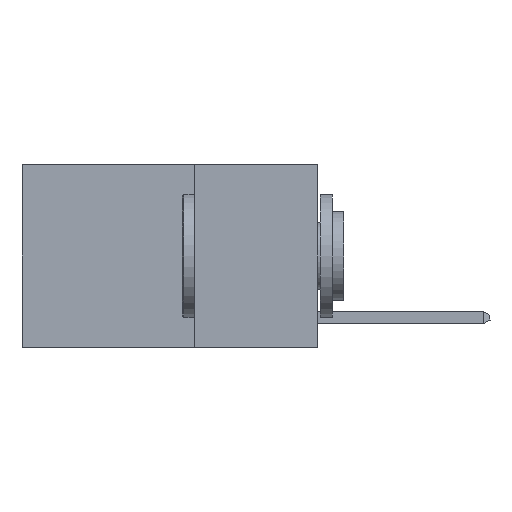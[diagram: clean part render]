
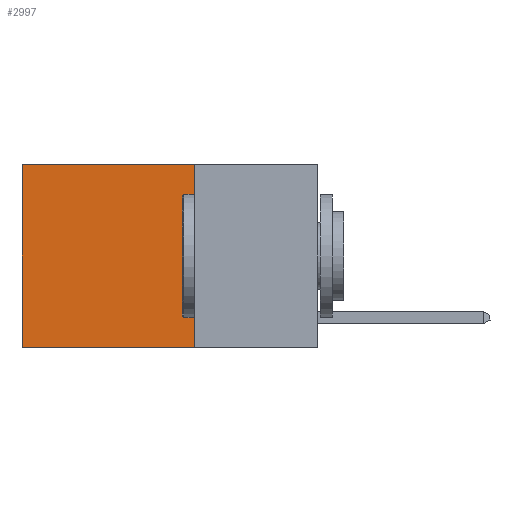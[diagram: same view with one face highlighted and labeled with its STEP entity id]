
A CAD part, left-side view. The second image highlights one B-rep face of the part: STEP entity #2997.
In plain terms, the highlighted planar face has unit normal (-1, 0, 0).
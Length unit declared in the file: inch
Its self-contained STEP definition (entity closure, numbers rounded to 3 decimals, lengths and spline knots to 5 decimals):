
#10 = FACE_OUTER_BOUND ( 'NONE', #14598, .T. ) ;
#168 = LINE ( 'NONE', #2548, #2207 ) ;
#1040 = CARTESIAN_POINT ( 'NONE',  ( 0.2625, 0.25, 0. ) ) ;
#2207 = VECTOR ( 'NONE', #10764, 39.37008 ) ;
#2548 = CARTESIAN_POINT ( 'NONE',  ( 0.2625, 0.25, 0. ) ) ;
#2997 = ADVANCED_FACE ( 'NONE', ( #10 ), #13399, .F. ) ;
#3444 = CARTESIAN_POINT ( 'NONE',  ( 0.2625, 0.25, -0.37 ) ) ;
#4680 = CARTESIAN_POINT ( 'NONE',  ( 0.2625, 0.6, 0. ) ) ;
#5190 = DIRECTION ( 'NONE',  ( 0., 0., -1. ) ) ;
#5893 = ORIENTED_EDGE ( 'NONE', *, *, #22824, .T. ) ;
#6298 = VERTEX_POINT ( 'NONE', #7119 ) ;
#7119 = CARTESIAN_POINT ( 'NONE',  ( 0.2625, 0.25, 0. ) ) ;
#7714 = ORIENTED_EDGE ( 'NONE', *, *, #14016, .T. ) ;
#8645 = CARTESIAN_POINT ( 'NONE',  ( 0.2625, 0.25, 0. ) ) ;
#9519 = VERTEX_POINT ( 'NONE', #22891 ) ;
#10262 = VECTOR ( 'NONE', #17862, 39.37008 ) ;
#10364 = ORIENTED_EDGE ( 'NONE', *, *, #26262, .F. ) ;
#10764 = DIRECTION ( 'NONE',  ( 0., 0., -1. ) ) ;
#11684 = CARTESIAN_POINT ( 'NONE',  ( 0.2625, 0.6, -0.37 ) ) ;
#13399 = PLANE ( 'NONE',  #26738 ) ;
#14016 = EDGE_CURVE ( 'NONE', #6298, #25260, #20219, .T. ) ;
#14598 = EDGE_LOOP ( 'NONE', ( #5893, #10364, #22666, #7714 ) ) ;
#17540 = DIRECTION ( 'NONE',  ( 1., 0., 0. ) ) ;
#17748 = VECTOR ( 'NONE', #23273, 39.37008 ) ;
#17862 = DIRECTION ( 'NONE',  ( 0., 1., 0. ) ) ;
#19584 = VECTOR ( 'NONE', #25146, 39.37008 ) ;
#20219 = LINE ( 'NONE', #8645, #19584 ) ;
#21230 = LINE ( 'NONE', #3444, #10262 ) ;
#22666 = ORIENTED_EDGE ( 'NONE', *, *, #25949, .F. ) ;
#22824 = EDGE_CURVE ( 'NONE', #25260, #23759, #23240, .T. ) ;
#22891 = CARTESIAN_POINT ( 'NONE',  ( 0.2625, 0.25, -0.37 ) ) ;
#23240 = LINE ( 'NONE', #4680, #17748 ) ;
#23273 = DIRECTION ( 'NONE',  ( 0., 0., -1. ) ) ;
#23759 = VERTEX_POINT ( 'NONE', #11684 ) ;
#25146 = DIRECTION ( 'NONE',  ( 0., 1., 0. ) ) ;
#25260 = VERTEX_POINT ( 'NONE', #26751 ) ;
#25949 = EDGE_CURVE ( 'NONE', #6298, #9519, #168, .T. ) ;
#26262 = EDGE_CURVE ( 'NONE', #9519, #23759, #21230, .T. ) ;
#26738 = AXIS2_PLACEMENT_3D ( 'NONE', #1040, #17540, #5190 ) ;
#26751 = CARTESIAN_POINT ( 'NONE',  ( 0.2625, 0.6, 0. ) ) ;
